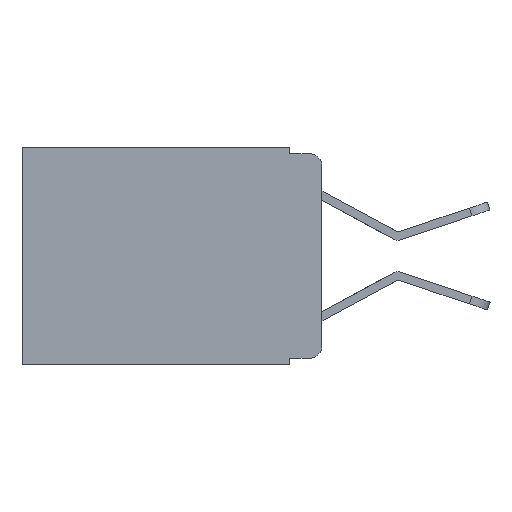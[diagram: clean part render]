
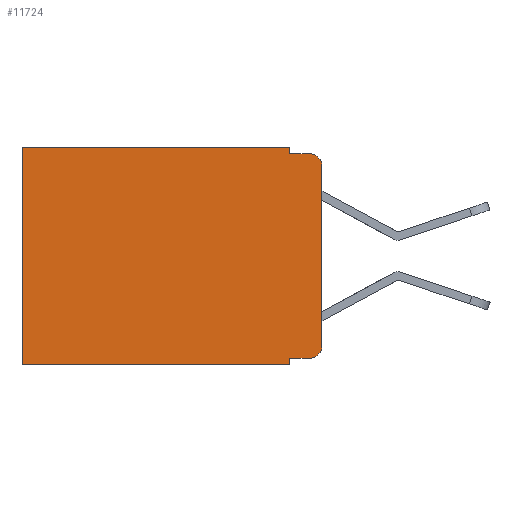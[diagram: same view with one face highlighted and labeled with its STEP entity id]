
A CAD part, left-side view. The second image highlights one B-rep face of the part: STEP entity #11724.
In plain terms, the highlighted planar face has unit normal (-1, 0, 0).
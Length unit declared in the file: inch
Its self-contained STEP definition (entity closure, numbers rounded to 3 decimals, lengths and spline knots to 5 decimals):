
#451 = VERTEX_POINT ( 'NONE', #4983 ) ;
#515 = ORIENTED_EDGE ( 'NONE', *, *, #5727, .T. ) ;
#518 = VERTEX_POINT ( 'NONE', #10696 ) ;
#592 = VERTEX_POINT ( 'NONE', #11903 ) ;
#593 = DIRECTION ( 'NONE',  ( 0., 0., -1. ) ) ;
#807 = LINE ( 'NONE', #12136, #5087 ) ;
#822 = CARTESIAN_POINT ( 'NONE',  ( 0.298, 0.051, 0. ) ) ;
#1422 = EDGE_CURVE ( 'NONE', #518, #6596, #11706, .T. ) ;
#1593 = EDGE_LOOP ( 'NONE', ( #8694, #3158, #6723, #11543, #515, #7425, #8773, #2677, #8155, #4045 ) ) ;
#1597 = VECTOR ( 'NONE', #6142, 39.37008 ) ;
#1630 = CARTESIAN_POINT ( 'NONE',  ( 0.298, 0., 0. ) ) ;
#1658 = EDGE_CURVE ( 'NONE', #9264, #3936, #3624, .T. ) ;
#2112 = CARTESIAN_POINT ( 'NONE',  ( 0.298, 0.02, -0.01 ) ) ;
#2161 = CARTESIAN_POINT ( 'NONE',  ( 0.298, 0.051, -0.01 ) ) ;
#2464 = CARTESIAN_POINT ( 'NONE',  ( 0.298, 0., 0. ) ) ;
#2505 = CARTESIAN_POINT ( 'NONE',  ( 0.298, 0.051, -0.333 ) ) ;
#2677 = ORIENTED_EDGE ( 'NONE', *, *, #1422, .F. ) ;
#2739 = DIRECTION ( 'NONE',  ( 0., 0., -1. ) ) ;
#2872 = DIRECTION ( 'NONE',  ( 0., 1., 0. ) ) ;
#2907 = DIRECTION ( 'NONE',  ( -1., 0., 0. ) ) ;
#2941 = LINE ( 'NONE', #2464, #6371 ) ;
#3158 = ORIENTED_EDGE ( 'NONE', *, *, #1658, .T. ) ;
#3512 = AXIS2_PLACEMENT_3D ( 'NONE', #12040, #4401, #11078 ) ;
#3565 = DIRECTION ( 'NONE',  ( 1., 0., 0. ) ) ;
#3624 = CIRCLE ( 'NONE', #3512, 0.02 ) ;
#3878 = VECTOR ( 'NONE', #10656, 39.37008 ) ;
#3936 = VERTEX_POINT ( 'NONE', #2112 ) ;
#4045 = ORIENTED_EDGE ( 'NONE', *, *, #12291, .T. ) ;
#4205 = CARTESIAN_POINT ( 'NONE',  ( 0.298, 0.051, -0.01 ) ) ;
#4280 = VERTEX_POINT ( 'NONE', #9920 ) ;
#4382 = LINE ( 'NONE', #5496, #9170 ) ;
#4401 = DIRECTION ( 'NONE',  ( -1., 0., 0. ) ) ;
#4499 = LINE ( 'NONE', #4814, #9443 ) ;
#4513 = DIRECTION ( 'NONE',  ( 0., 0., -1. ) ) ;
#4812 = FACE_OUTER_BOUND ( 'NONE', #1593, .T. ) ;
#4814 = CARTESIAN_POINT ( 'NONE',  ( 0.298, 0., -0.343 ) ) ;
#4983 = CARTESIAN_POINT ( 'NONE',  ( 0.298, 0., -0.313 ) ) ;
#5087 = VECTOR ( 'NONE', #6528, 39.37008 ) ;
#5369 = EDGE_CURVE ( 'NONE', #518, #10886, #5920, .T. ) ;
#5496 = CARTESIAN_POINT ( 'NONE',  ( 0.298, 0.473, 0. ) ) ;
#5727 = EDGE_CURVE ( 'NONE', #8895, #592, #807, .T. ) ;
#5759 = VERTEX_POINT ( 'NONE', #2161 ) ;
#5920 = LINE ( 'NONE', #2505, #10416 ) ;
#5975 = LINE ( 'NONE', #8744, #3878 ) ;
#6142 = DIRECTION ( 'NONE',  ( 0., -1., 0. ) ) ;
#6217 = LINE ( 'NONE', #4205, #1597 ) ;
#6371 = VECTOR ( 'NONE', #593, 39.37008 ) ;
#6419 = PLANE ( 'NONE',  #10813 ) ;
#6528 = DIRECTION ( 'NONE',  ( 0., 1., 0. ) ) ;
#6596 = VERTEX_POINT ( 'NONE', #9857 ) ;
#6723 = ORIENTED_EDGE ( 'NONE', *, *, #9469, .F. ) ;
#6778 = EDGE_CURVE ( 'NONE', #8895, #5759, #5975, .T. ) ;
#6894 = AXIS2_PLACEMENT_3D ( 'NONE', #9563, #2907, #9610 ) ;
#7173 = CARTESIAN_POINT ( 'NONE',  ( 0.298, 0.051, 0. ) ) ;
#7425 = ORIENTED_EDGE ( 'NONE', *, *, #10877, .T. ) ;
#8155 = ORIENTED_EDGE ( 'NONE', *, *, #5369, .T. ) ;
#8239 = CIRCLE ( 'NONE', #6894, 0.02 ) ;
#8442 = CARTESIAN_POINT ( 'NONE',  ( 0.298, 0., -0.03 ) ) ;
#8694 = ORIENTED_EDGE ( 'NONE', *, *, #9414, .F. ) ;
#8744 = CARTESIAN_POINT ( 'NONE',  ( 0.298, 0.051, 0. ) ) ;
#8773 = ORIENTED_EDGE ( 'NONE', *, *, #11727, .F. ) ;
#8895 = VERTEX_POINT ( 'NONE', #7173 ) ;
#9170 = VECTOR ( 'NONE', #11997, 39.37008 ) ;
#9264 = VERTEX_POINT ( 'NONE', #8442 ) ;
#9326 = CARTESIAN_POINT ( 'NONE',  ( 0.298, 0.02, -0.333 ) ) ;
#9414 = EDGE_CURVE ( 'NONE', #9264, #451, #2941, .T. ) ;
#9443 = VECTOR ( 'NONE', #2872, 39.37008 ) ;
#9469 = EDGE_CURVE ( 'NONE', #5759, #3936, #6217, .T. ) ;
#9563 = CARTESIAN_POINT ( 'NONE',  ( 0.298, 0.02, -0.313 ) ) ;
#9610 = DIRECTION ( 'NONE',  ( 0., 0., -1. ) ) ;
#9857 = CARTESIAN_POINT ( 'NONE',  ( 0.298, 0.051, -0.343 ) ) ;
#9920 = CARTESIAN_POINT ( 'NONE',  ( 0.298, 0.473, -0.343 ) ) ;
#10416 = VECTOR ( 'NONE', #11108, 39.37008 ) ;
#10656 = DIRECTION ( 'NONE',  ( 0., 0., -1. ) ) ;
#10690 = VECTOR ( 'NONE', #2739, 39.37008 ) ;
#10696 = CARTESIAN_POINT ( 'NONE',  ( 0.298, 0.051, -0.333 ) ) ;
#10813 = AXIS2_PLACEMENT_3D ( 'NONE', #1630, #3565, #4513 ) ;
#10877 = EDGE_CURVE ( 'NONE', #592, #4280, #4382, .T. ) ;
#10886 = VERTEX_POINT ( 'NONE', #9326 ) ;
#11078 = DIRECTION ( 'NONE',  ( 0., 0., -1. ) ) ;
#11108 = DIRECTION ( 'NONE',  ( 0., -1., 0. ) ) ;
#11543 = ORIENTED_EDGE ( 'NONE', *, *, #6778, .F. ) ;
#11706 = LINE ( 'NONE', #822, #10690 ) ;
#11724 = ADVANCED_FACE ( 'NONE', ( #4812 ), #6419, .F. ) ;
#11727 = EDGE_CURVE ( 'NONE', #6596, #4280, #4499, .T. ) ;
#11903 = CARTESIAN_POINT ( 'NONE',  ( 0.298, 0.473, 0. ) ) ;
#11997 = DIRECTION ( 'NONE',  ( 0., 0., -1. ) ) ;
#12040 = CARTESIAN_POINT ( 'NONE',  ( 0.298, 0.02, -0.03 ) ) ;
#12136 = CARTESIAN_POINT ( 'NONE',  ( 0.298, 0., 0. ) ) ;
#12291 = EDGE_CURVE ( 'NONE', #10886, #451, #8239, .T. ) ;
